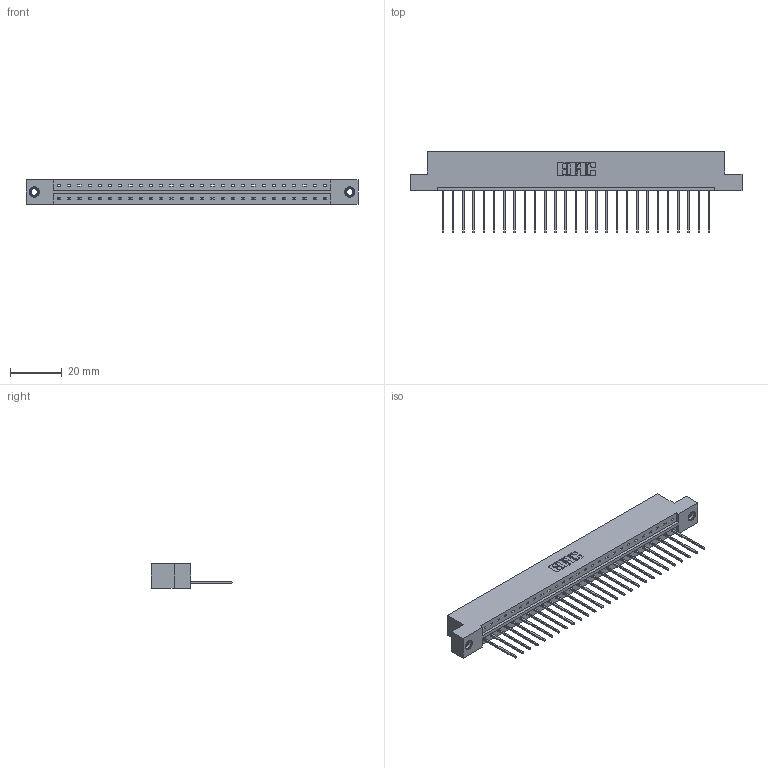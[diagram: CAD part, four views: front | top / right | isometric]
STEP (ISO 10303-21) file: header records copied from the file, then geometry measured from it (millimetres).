
FILE_DESCRIPTION (( 'STEP AP203' ), '1' );
FILE_NAME ('833-027-542-107.STEP', '2020-06-02T06:55:17', ( '' ), ( '' ), 'SwSTEP 2.0', 'SolidWorks 2020', '' );
FILE_SCHEMA (( 'CONFIG_CONTROL_DESIGN' ));
Length unit declared in the file: inch
Products named in the file (4): 833 Part_Flush - .156 Dia - TI; 345-250-001_345-250-005-103; 345-292-001_345-293-142; 833-027-542-107
Assembly tree (30 placements, depth 2):
  833-027-542-107
    833 Part_Flush - .156 Dia - TI
    345-292-001_345-293-142  x27
    345-250-001_345-250-005-103  x2
Bounding box: 128.52 x 31.63 x 9.4 mm (x, y, z)
Volume: 12850.7 mm3; surface area: 14239.1 mm2
Topology: 30 solids, 30 shells, 1740 faces, 5199 edges, 3422 vertices
Faces by surface type: plane 1236, cylinder 488, cone 12, torus 4
Entity records: 19650 total; most frequent: CARTESIAN_POINT 3374, ORIENTED_EDGE 3330, DIRECTION 2909, EDGE_CURVE 1665, VECTOR 1517, LINE 1517, VERTEX_POINT 1104, AXIS2_PLACEMENT_3D 696
